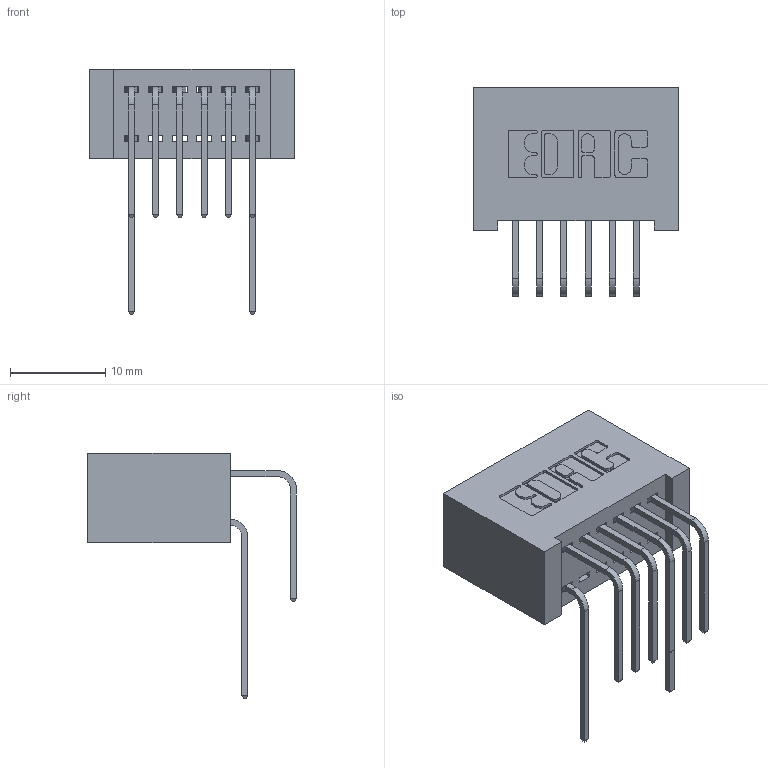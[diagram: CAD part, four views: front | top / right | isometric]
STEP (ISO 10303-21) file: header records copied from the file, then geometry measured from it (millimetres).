
FILE_DESCRIPTION (( 'STEP AP203' ), '1' );
FILE_NAME ('392-012-558-201.STEP', '2018-08-14T22:36:03', ( '' ), ( '' ), 'SwSTEP 2.0', 'SolidWorks 2016', '' );
FILE_SCHEMA (( 'CONFIG_CONTROL_DESIGN' ));
Length unit declared in the file: inch
Products named in the file (4): 342 Part_Lugless; 345-292-001_558 559 Tail - 1; 345-292-001_558 Tail - 2; 392-012-558-201
Assembly tree (9 placements, depth 2):
  392-012-558-201
    342 Part_Lugless
    345-292-001_558 559 Tail - 1  x2
    345-292-001_558 Tail - 2  x6
Bounding box: 21.49 x 21.91 x 25.78 mm (x, y, z)
Volume: 2210 mm3; surface area: 3166.3 mm2
Topology: 9 solids, 9 shells, 558 faces, 1647 edges, 1086 vertices
Faces by surface type: plane 390, cylinder 168
Entity records: 9763 total; most frequent: CARTESIAN_POINT 1725, ORIENTED_EDGE 1614, DIRECTION 1507, EDGE_CURVE 807, VECTOR 647, LINE 647, VERTEX_POINT 534, AXIS2_PLACEMENT_3D 430
